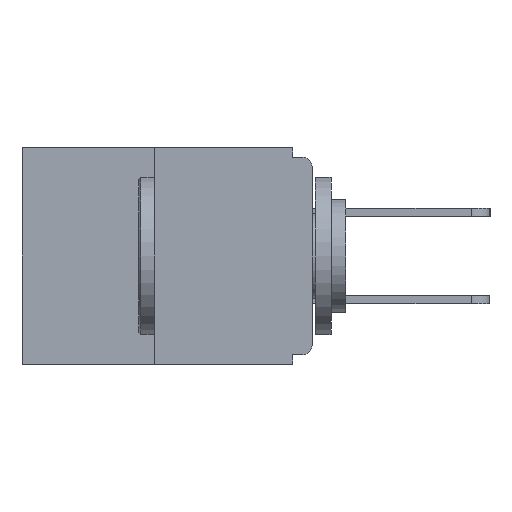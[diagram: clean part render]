
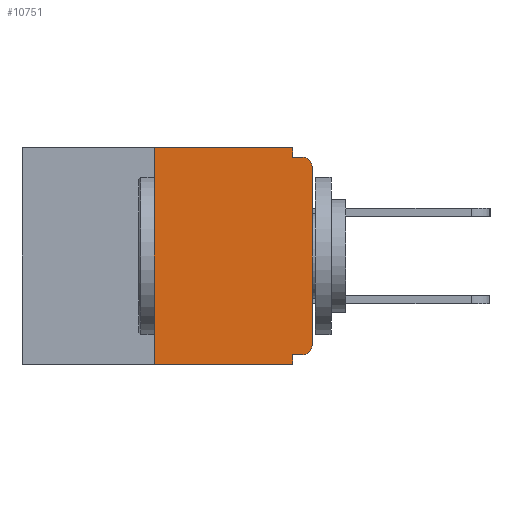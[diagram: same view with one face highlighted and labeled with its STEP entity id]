
A CAD part, left-side view. The second image highlights one B-rep face of the part: STEP entity #10751.
In plain terms, the highlighted planar face has unit normal (-1, 0, 0).
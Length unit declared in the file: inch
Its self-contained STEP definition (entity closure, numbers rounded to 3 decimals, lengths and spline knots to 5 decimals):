
#473 = DIRECTION ( 'NONE',  ( 0., -1., 0. ) ) ;
#680 = VECTOR ( 'NONE', #2537, 39.37008 ) ;
#1670 = LINE ( 'NONE', #2529, #15867 ) ;
#1763 = VERTEX_POINT ( 'NONE', #7897 ) ;
#1769 = VERTEX_POINT ( 'NONE', #22624 ) ;
#2529 = CARTESIAN_POINT ( 'NONE',  ( 0., 0.46, -0.343 ) ) ;
#2537 = DIRECTION ( 'NONE',  ( 0., 1., 0. ) ) ;
#2808 = VECTOR ( 'NONE', #473, 39.37008 ) ;
#3039 = CARTESIAN_POINT ( 'NONE',  ( 0., 0., 0. ) ) ;
#3571 = ORIENTED_EDGE ( 'NONE', *, *, #16028, .F. ) ;
#3793 = EDGE_CURVE ( 'NONE', #1769, #22106, #1670, .T. ) ;
#4040 = CARTESIAN_POINT ( 'NONE',  ( 0., 0.015, -0.313 ) ) ;
#4222 = VERTEX_POINT ( 'NONE', #14134 ) ;
#4405 = DIRECTION ( 'NONE',  ( 0., -1., 0. ) ) ;
#4502 = EDGE_CURVE ( 'NONE', #11053, #20446, #12867, .T. ) ;
#4834 = EDGE_CURVE ( 'NONE', #11978, #22106, #5924, .T. ) ;
#4917 = CARTESIAN_POINT ( 'NONE',  ( 0., 0.031, -0.343 ) ) ;
#5194 = DIRECTION ( 'NONE',  ( 0., 0., 1. ) ) ;
#5737 = CARTESIAN_POINT ( 'NONE',  ( 0., 0.031, -0.015 ) ) ;
#5913 = VECTOR ( 'NONE', #25379, 39.37008 ) ;
#5924 = LINE ( 'NONE', #21053, #15807 ) ;
#5933 = CIRCLE ( 'NONE', #14503, 0.015 ) ;
#6177 = DIRECTION ( 'NONE',  ( 0., 0., -1. ) ) ;
#6402 = ORIENTED_EDGE ( 'NONE', *, *, #8878, .T. ) ;
#6538 = DIRECTION ( 'NONE',  ( 0., 0., -1. ) ) ;
#6635 = PLANE ( 'NONE',  #18314 ) ;
#6708 = CARTESIAN_POINT ( 'NONE',  ( 0., 0.46, 0. ) ) ;
#7762 = VECTOR ( 'NONE', #26365, 39.37008 ) ;
#7897 = CARTESIAN_POINT ( 'NONE',  ( 0., 0.015, -0.328 ) ) ;
#8107 = ORIENTED_EDGE ( 'NONE', *, *, #16894, .T. ) ;
#8169 = CARTESIAN_POINT ( 'NONE',  ( 0., 0.031, -0.328 ) ) ;
#8878 = EDGE_CURVE ( 'NONE', #1763, #11053, #24840, .T. ) ;
#9307 = LINE ( 'NONE', #24008, #680 ) ;
#10143 = DIRECTION ( 'NONE',  ( 0., 0., -1. ) ) ;
#10250 = DIRECTION ( 'NONE',  ( -1., 0., 0. ) ) ;
#10566 = ORIENTED_EDGE ( 'NONE', *, *, #25195, .F. ) ;
#10751 = ADVANCED_FACE ( 'NONE', ( #21779 ), #6635, .F. ) ;
#11053 = VERTEX_POINT ( 'NONE', #26767 ) ;
#11185 = EDGE_CURVE ( 'NONE', #12708, #20031, #17819, .T. ) ;
#11711 = CARTESIAN_POINT ( 'NONE',  ( 0., 0.015, -0.015 ) ) ;
#11978 = VERTEX_POINT ( 'NONE', #8169 ) ;
#12708 = VERTEX_POINT ( 'NONE', #5737 ) ;
#12867 = LINE ( 'NONE', #3039, #18845 ) ;
#13309 = EDGE_CURVE ( 'NONE', #1769, #26039, #17404, .T. ) ;
#14134 = CARTESIAN_POINT ( 'NONE',  ( 0., 0.031, 0. ) ) ;
#14144 = CARTESIAN_POINT ( 'NONE',  ( 0., 0., -0.03 ) ) ;
#14503 = AXIS2_PLACEMENT_3D ( 'NONE', #21426, #21602, #25729 ) ;
#14554 = AXIS2_PLACEMENT_3D ( 'NONE', #4040, #10250, #10143 ) ;
#14619 = ORIENTED_EDGE ( 'NONE', *, *, #24672, .F. ) ;
#14947 = CARTESIAN_POINT ( 'NONE',  ( 0., 0.46, 0. ) ) ;
#15112 = DIRECTION ( 'NONE',  ( 1., 0., 0. ) ) ;
#15602 = CARTESIAN_POINT ( 'NONE',  ( 0., 0.031, 0. ) ) ;
#15807 = VECTOR ( 'NONE', #6177, 39.37008 ) ;
#15867 = VECTOR ( 'NONE', #4405, 39.37008 ) ;
#16028 = EDGE_CURVE ( 'NONE', #1763, #11978, #9307, .T. ) ;
#16550 = ORIENTED_EDGE ( 'NONE', *, *, #13309, .F. ) ;
#16815 = CARTESIAN_POINT ( 'NONE',  ( 0., 0.25, 0. ) ) ;
#16894 = EDGE_CURVE ( 'NONE', #20446, #20031, #5933, .T. ) ;
#17404 = LINE ( 'NONE', #16815, #26582 ) ;
#17819 = LINE ( 'NONE', #22906, #5913 ) ;
#18314 = AXIS2_PLACEMENT_3D ( 'NONE', #14947, #15112, #6538 ) ;
#18335 = CARTESIAN_POINT ( 'NONE',  ( 0., 0.25, 0. ) ) ;
#18845 = VECTOR ( 'NONE', #5194, 39.37008 ) ;
#19010 = LINE ( 'NONE', #15602, #7762 ) ;
#19941 = ORIENTED_EDGE ( 'NONE', *, *, #4834, .F. ) ;
#20031 = VERTEX_POINT ( 'NONE', #11711 ) ;
#20151 = ORIENTED_EDGE ( 'NONE', *, *, #4502, .T. ) ;
#20319 = LINE ( 'NONE', #6708, #2808 ) ;
#20446 = VERTEX_POINT ( 'NONE', #14144 ) ;
#21053 = CARTESIAN_POINT ( 'NONE',  ( 0., 0.031, -0.343 ) ) ;
#21417 = EDGE_LOOP ( 'NONE', ( #14619, #16550, #24170, #19941, #3571, #6402, #20151, #8107, #25455, #10566 ) ) ;
#21426 = CARTESIAN_POINT ( 'NONE',  ( 0., 0.015, -0.03 ) ) ;
#21602 = DIRECTION ( 'NONE',  ( -1., 0., 0. ) ) ;
#21779 = FACE_OUTER_BOUND ( 'NONE', #21417, .T. ) ;
#22106 = VERTEX_POINT ( 'NONE', #4917 ) ;
#22624 = CARTESIAN_POINT ( 'NONE',  ( 0., 0.25, -0.343 ) ) ;
#22906 = CARTESIAN_POINT ( 'NONE',  ( 0., 0., -0.015 ) ) ;
#23142 = DIRECTION ( 'NONE',  ( 0., 0., 1. ) ) ;
#24008 = CARTESIAN_POINT ( 'NONE',  ( 0., 0., -0.328 ) ) ;
#24170 = ORIENTED_EDGE ( 'NONE', *, *, #3793, .T. ) ;
#24672 = EDGE_CURVE ( 'NONE', #26039, #4222, #20319, .T. ) ;
#24840 = CIRCLE ( 'NONE', #14554, 0.015 ) ;
#25195 = EDGE_CURVE ( 'NONE', #4222, #12708, #19010, .T. ) ;
#25379 = DIRECTION ( 'NONE',  ( 0., -1., 0. ) ) ;
#25455 = ORIENTED_EDGE ( 'NONE', *, *, #11185, .F. ) ;
#25729 = DIRECTION ( 'NONE',  ( 0., 0., -1. ) ) ;
#26039 = VERTEX_POINT ( 'NONE', #18335 ) ;
#26365 = DIRECTION ( 'NONE',  ( 0., 0., -1. ) ) ;
#26582 = VECTOR ( 'NONE', #23142, 39.37008 ) ;
#26767 = CARTESIAN_POINT ( 'NONE',  ( 0., 0., -0.313 ) ) ;
